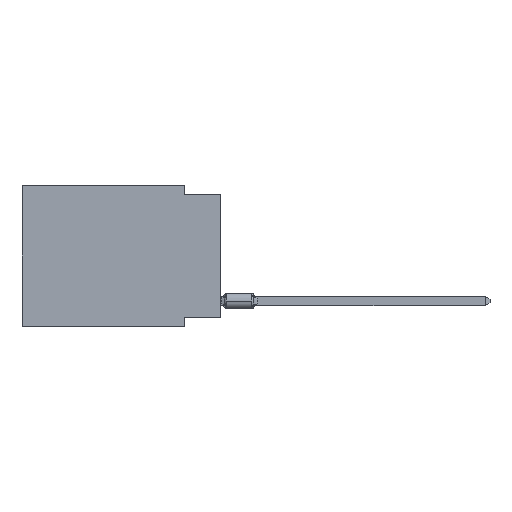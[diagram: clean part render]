
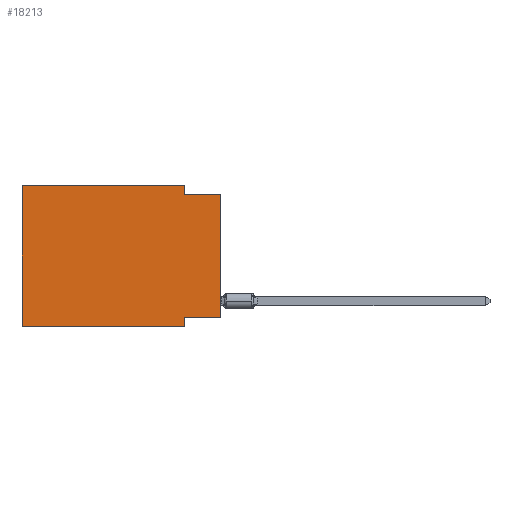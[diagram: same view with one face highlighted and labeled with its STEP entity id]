
A CAD part, left-side view. The second image highlights one B-rep face of the part: STEP entity #18213.
In plain terms, the highlighted planar face has unit normal (-1, 0, 0).
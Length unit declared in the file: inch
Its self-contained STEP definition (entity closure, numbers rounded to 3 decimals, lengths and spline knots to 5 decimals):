
#27 = VERTEX_POINT ( 'NONE', #16304 ) ;
#374 = ORIENTED_EDGE ( 'NONE', *, *, #15220, .F. ) ;
#527 = CARTESIAN_POINT ( 'NONE',  ( 0., 0.1, -0.025 ) ) ;
#687 = ORIENTED_EDGE ( 'NONE', *, *, #5019, .T. ) ;
#990 = DIRECTION ( 'NONE',  ( 0., -1., 0. ) ) ;
#1151 = ORIENTED_EDGE ( 'NONE', *, *, #19134, .F. ) ;
#1363 = DIRECTION ( 'NONE',  ( 0., -1., 0. ) ) ;
#1543 = VECTOR ( 'NONE', #19588, 39.37008 ) ;
#2580 = CARTESIAN_POINT ( 'NONE',  ( 0., 0.1, -0.365 ) ) ;
#2791 = LINE ( 'NONE', #12566, #6904 ) ;
#2971 = LINE ( 'NONE', #9364, #6170 ) ;
#3283 = CARTESIAN_POINT ( 'NONE',  ( 0., 0.1, 0. ) ) ;
#3440 = DIRECTION ( 'NONE',  ( 0., 0., 1. ) ) ;
#3710 = VERTEX_POINT ( 'NONE', #8992 ) ;
#3927 = ORIENTED_EDGE ( 'NONE', *, *, #12474, .F. ) ;
#4161 = EDGE_LOOP ( 'NONE', ( #687, #4202, #9495, #3927, #374, #17997, #1151, #4961 ) ) ;
#4202 = ORIENTED_EDGE ( 'NONE', *, *, #14901, .F. ) ;
#4309 = VERTEX_POINT ( 'NONE', #527 ) ;
#4961 = ORIENTED_EDGE ( 'NONE', *, *, #14925, .F. ) ;
#5019 = EDGE_CURVE ( 'NONE', #13808, #10551, #6418, .T. ) ;
#5766 = PLANE ( 'NONE',  #12750 ) ;
#5786 = LINE ( 'NONE', #7273, #12620 ) ;
#6050 = CARTESIAN_POINT ( 'NONE',  ( 0., 0.55, -0.39 ) ) ;
#6155 = DIRECTION ( 'NONE',  ( 0., -1., 0. ) ) ;
#6156 = CARTESIAN_POINT ( 'NONE',  ( 0., 0.55, -0.39 ) ) ;
#6170 = VECTOR ( 'NONE', #1363, 39.37008 ) ;
#6418 = LINE ( 'NONE', #12809, #18071 ) ;
#6533 = EDGE_CURVE ( 'NONE', #11394, #4309, #2791, .T. ) ;
#6904 = VECTOR ( 'NONE', #19056, 39.37008 ) ;
#7273 = CARTESIAN_POINT ( 'NONE',  ( 0., 0., -0.025 ) ) ;
#7353 = DIRECTION ( 'NONE',  ( 0., 0., -1. ) ) ;
#7376 = CARTESIAN_POINT ( 'NONE',  ( 0., 0., -0.365 ) ) ;
#8066 = CARTESIAN_POINT ( 'NONE',  ( 0., 0., -0.365 ) ) ;
#8885 = VECTOR ( 'NONE', #12475, 39.37008 ) ;
#8940 = LINE ( 'NONE', #9822, #12984 ) ;
#8992 = CARTESIAN_POINT ( 'NONE',  ( 0., 0.55, 0. ) ) ;
#9364 = CARTESIAN_POINT ( 'NONE',  ( 0., 0.55, 0. ) ) ;
#9395 = DIRECTION ( 'NONE',  ( 1., 0., 0. ) ) ;
#9495 = ORIENTED_EDGE ( 'NONE', *, *, #6533, .F. ) ;
#9822 = CARTESIAN_POINT ( 'NONE',  ( 0., 0.55, 0. ) ) ;
#10274 = VECTOR ( 'NONE', #6155, 39.37008 ) ;
#10551 = VERTEX_POINT ( 'NONE', #12690 ) ;
#11394 = VERTEX_POINT ( 'NONE', #3283 ) ;
#12259 = LINE ( 'NONE', #7376, #8885 ) ;
#12474 = EDGE_CURVE ( 'NONE', #3710, #11394, #2971, .T. ) ;
#12475 = DIRECTION ( 'NONE',  ( 0., 1., 0. ) ) ;
#12566 = CARTESIAN_POINT ( 'NONE',  ( 0., 0.1, 0. ) ) ;
#12620 = VECTOR ( 'NONE', #990, 39.37008 ) ;
#12690 = CARTESIAN_POINT ( 'NONE',  ( 0., 0., -0.025 ) ) ;
#12750 = AXIS2_PLACEMENT_3D ( 'NONE', #18949, #9395, #7353 ) ;
#12809 = CARTESIAN_POINT ( 'NONE',  ( 0., 0., 0. ) ) ;
#12984 = VECTOR ( 'NONE', #15418, 39.37008 ) ;
#13656 = VERTEX_POINT ( 'NONE', #6156 ) ;
#13808 = VERTEX_POINT ( 'NONE', #8066 ) ;
#14051 = EDGE_CURVE ( 'NONE', #13656, #27, #15629, .T. ) ;
#14510 = LINE ( 'NONE', #17809, #1543 ) ;
#14901 = EDGE_CURVE ( 'NONE', #4309, #10551, #5786, .T. ) ;
#14925 = EDGE_CURVE ( 'NONE', #13808, #18233, #12259, .T. ) ;
#15220 = EDGE_CURVE ( 'NONE', #13656, #3710, #8940, .T. ) ;
#15418 = DIRECTION ( 'NONE',  ( 0., 0., 1. ) ) ;
#15629 = LINE ( 'NONE', #6050, #10274 ) ;
#16304 = CARTESIAN_POINT ( 'NONE',  ( 0., 0.1, -0.39 ) ) ;
#17809 = CARTESIAN_POINT ( 'NONE',  ( 0., 0.1, -0.39 ) ) ;
#17997 = ORIENTED_EDGE ( 'NONE', *, *, #14051, .T. ) ;
#18071 = VECTOR ( 'NONE', #3440, 39.37008 ) ;
#18213 = ADVANCED_FACE ( 'NONE', ( #20421 ), #5766, .F. ) ;
#18233 = VERTEX_POINT ( 'NONE', #2580 ) ;
#18949 = CARTESIAN_POINT ( 'NONE',  ( 0., 0.55, 0. ) ) ;
#19056 = DIRECTION ( 'NONE',  ( 0., 0., -1. ) ) ;
#19134 = EDGE_CURVE ( 'NONE', #18233, #27, #14510, .T. ) ;
#19588 = DIRECTION ( 'NONE',  ( 0., 0., -1. ) ) ;
#20421 = FACE_OUTER_BOUND ( 'NONE', #4161, .T. ) ;
